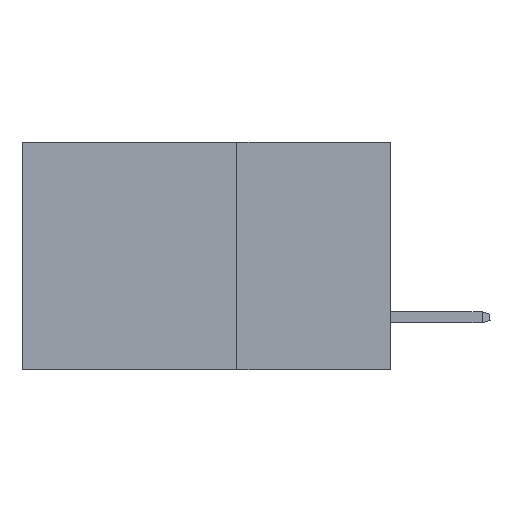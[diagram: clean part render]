
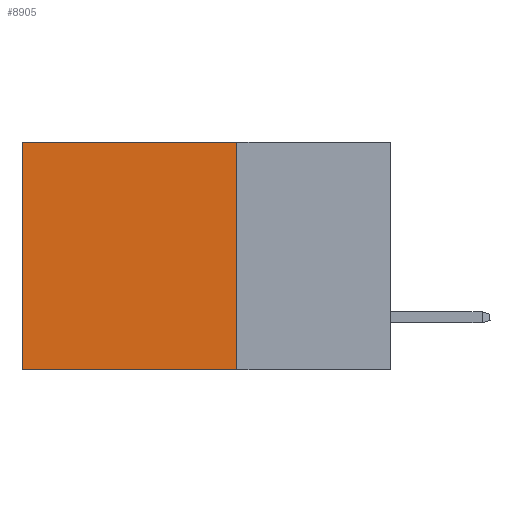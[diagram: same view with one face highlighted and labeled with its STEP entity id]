
A CAD part, left-side view. The second image highlights one B-rep face of the part: STEP entity #8905.
In plain terms, the highlighted planar face has unit normal (-1, 0, 0).
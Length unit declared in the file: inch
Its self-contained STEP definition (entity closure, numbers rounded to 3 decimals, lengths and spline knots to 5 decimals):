
#308 = CARTESIAN_POINT ( 'NONE',  ( 0.2875, 0.6, -0.37 ) ) ;
#436 = CARTESIAN_POINT ( 'NONE',  ( 0.2875, 0.6, 0. ) ) ;
#630 = VERTEX_POINT ( 'NONE', #436 ) ;
#767 = CARTESIAN_POINT ( 'NONE',  ( 0.2875, 0.25, 0. ) ) ;
#920 = DIRECTION ( 'NONE',  ( 0., 0., -1. ) ) ;
#958 = EDGE_CURVE ( 'NONE', #3388, #6511, #7849, .T. ) ;
#964 = EDGE_CURVE ( 'NONE', #9237, #3388, #5360, .T. ) ;
#1036 = ORIENTED_EDGE ( 'NONE', *, *, #958, .F. ) ;
#1923 = EDGE_LOOP ( 'NONE', ( #7734, #1036, #4618, #2891 ) ) ;
#2142 = CARTESIAN_POINT ( 'NONE',  ( 0.2875, 0.25, 0. ) ) ;
#2891 = ORIENTED_EDGE ( 'NONE', *, *, #3588, .T. ) ;
#2954 = VECTOR ( 'NONE', #7683, 39.37008 ) ;
#3388 = VERTEX_POINT ( 'NONE', #9119 ) ;
#3588 = EDGE_CURVE ( 'NONE', #9237, #630, #9776, .T. ) ;
#3777 = DIRECTION ( 'NONE',  ( 0., 1., 0. ) ) ;
#4618 = ORIENTED_EDGE ( 'NONE', *, *, #964, .F. ) ;
#5360 = LINE ( 'NONE', #767, #2954 ) ;
#5435 = DIRECTION ( 'NONE',  ( 0., 0., -1. ) ) ;
#5491 = VECTOR ( 'NONE', #6239, 39.37008 ) ;
#6137 = CARTESIAN_POINT ( 'NONE',  ( 0.2875, 0.25, 0. ) ) ;
#6239 = DIRECTION ( 'NONE',  ( 0., 1., 0. ) ) ;
#6354 = EDGE_CURVE ( 'NONE', #630, #6511, #6533, .T. ) ;
#6511 = VERTEX_POINT ( 'NONE', #308 ) ;
#6533 = LINE ( 'NONE', #7871, #6782 ) ;
#6554 = FACE_OUTER_BOUND ( 'NONE', #1923, .T. ) ;
#6782 = VECTOR ( 'NONE', #920, 39.37008 ) ;
#6895 = CARTESIAN_POINT ( 'NONE',  ( 0.2875, 0.25, 0. ) ) ;
#7683 = DIRECTION ( 'NONE',  ( 0., 0., -1. ) ) ;
#7734 = ORIENTED_EDGE ( 'NONE', *, *, #6354, .T. ) ;
#7849 = LINE ( 'NONE', #8601, #5491 ) ;
#7871 = CARTESIAN_POINT ( 'NONE',  ( 0.2875, 0.6, 0. ) ) ;
#7900 = AXIS2_PLACEMENT_3D ( 'NONE', #6137, #8401, #5435 ) ;
#8401 = DIRECTION ( 'NONE',  ( 1., 0., 0. ) ) ;
#8582 = PLANE ( 'NONE',  #7900 ) ;
#8601 = CARTESIAN_POINT ( 'NONE',  ( 0.2875, 0.25, -0.37 ) ) ;
#8905 = ADVANCED_FACE ( 'NONE', ( #6554 ), #8582, .F. ) ;
#8909 = VECTOR ( 'NONE', #3777, 39.37008 ) ;
#9119 = CARTESIAN_POINT ( 'NONE',  ( 0.2875, 0.25, -0.37 ) ) ;
#9237 = VERTEX_POINT ( 'NONE', #6895 ) ;
#9776 = LINE ( 'NONE', #2142, #8909 ) ;
